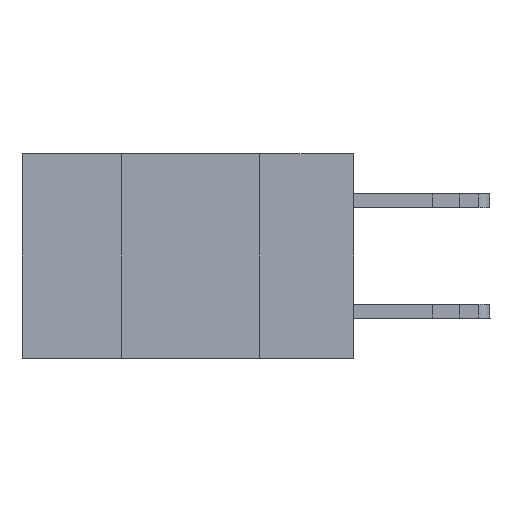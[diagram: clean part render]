
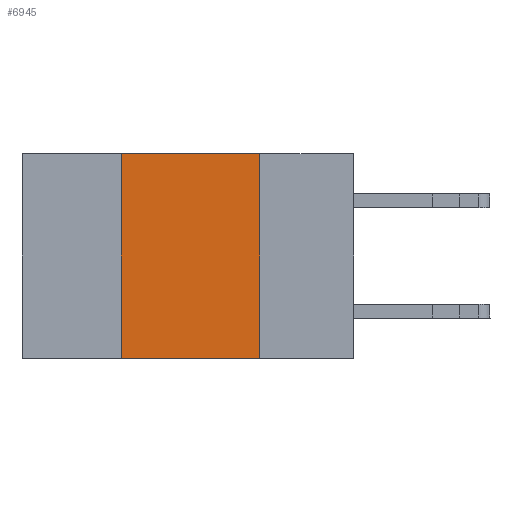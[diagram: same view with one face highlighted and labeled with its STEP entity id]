
A CAD part, left-side view. The second image highlights one B-rep face of the part: STEP entity #6945.
In plain terms, the highlighted planar face has unit normal (-1, 0, 0).
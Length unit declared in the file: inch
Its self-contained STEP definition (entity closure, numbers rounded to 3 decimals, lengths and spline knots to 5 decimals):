
#1055 = ORIENTED_EDGE ( 'NONE', *, *, #6135, .F. ) ;
#1481 = CARTESIAN_POINT ( 'NONE',  ( 0., 0.42, 0. ) ) ;
#1573 = DIRECTION ( 'NONE',  ( 0., 0., 1. ) ) ;
#2128 = DIRECTION ( 'NONE',  ( 0., 0., -1. ) ) ;
#2365 = PLANE ( 'NONE',  #15546 ) ;
#3663 = EDGE_CURVE ( 'NONE', #11657, #14002, #18799, .T. ) ;
#3861 = DIRECTION ( 'NONE',  ( 0., 0., -1. ) ) ;
#4919 = VERTEX_POINT ( 'NONE', #12031 ) ;
#6135 = EDGE_CURVE ( 'NONE', #14002, #4919, #16104, .T. ) ;
#6945 = ADVANCED_FACE ( 'NONE', ( #17276 ), #2365, .F. ) ;
#7197 = LINE ( 'NONE', #10608, #14643 ) ;
#7271 = ORIENTED_EDGE ( 'NONE', *, *, #3663, .F. ) ;
#7960 = VECTOR ( 'NONE', #16594, 39.37008 ) ;
#9075 = LINE ( 'NONE', #12852, #12044 ) ;
#9077 = EDGE_CURVE ( 'NONE', #13893, #11657, #7197, .T. ) ;
#9444 = EDGE_CURVE ( 'NONE', #13893, #4919, #9075, .T. ) ;
#9896 = DIRECTION ( 'NONE',  ( 0., -1., 0. ) ) ;
#10608 = CARTESIAN_POINT ( 'NONE',  ( 0., 0.42, 0. ) ) ;
#11132 = CARTESIAN_POINT ( 'NONE',  ( 0., 0.17, 0. ) ) ;
#11228 = VECTOR ( 'NONE', #2128, 39.37008 ) ;
#11385 = EDGE_LOOP ( 'NONE', ( #1055, #7271, #14712, #11914 ) ) ;
#11657 = VERTEX_POINT ( 'NONE', #1481 ) ;
#11914 = ORIENTED_EDGE ( 'NONE', *, *, #9444, .T. ) ;
#12031 = CARTESIAN_POINT ( 'NONE',  ( 0., 0.17, -0.37 ) ) ;
#12044 = VECTOR ( 'NONE', #9896, 39.37008 ) ;
#12844 = DIRECTION ( 'NONE',  ( 1., 0., 0. ) ) ;
#12852 = CARTESIAN_POINT ( 'NONE',  ( 0., 0.6, -0.37 ) ) ;
#13893 = VERTEX_POINT ( 'NONE', #16027 ) ;
#14002 = VERTEX_POINT ( 'NONE', #14793 ) ;
#14643 = VECTOR ( 'NONE', #1573, 39.37008 ) ;
#14712 = ORIENTED_EDGE ( 'NONE', *, *, #9077, .F. ) ;
#14793 = CARTESIAN_POINT ( 'NONE',  ( 0., 0.17, 0. ) ) ;
#15546 = AXIS2_PLACEMENT_3D ( 'NONE', #18739, #12844, #3861 ) ;
#15784 = CARTESIAN_POINT ( 'NONE',  ( 0., 0.6, 0. ) ) ;
#16027 = CARTESIAN_POINT ( 'NONE',  ( 0., 0.42, -0.37 ) ) ;
#16104 = LINE ( 'NONE', #11132, #11228 ) ;
#16594 = DIRECTION ( 'NONE',  ( 0., -1., 0. ) ) ;
#17276 = FACE_OUTER_BOUND ( 'NONE', #11385, .T. ) ;
#18739 = CARTESIAN_POINT ( 'NONE',  ( 0., 0.6, 0. ) ) ;
#18799 = LINE ( 'NONE', #15784, #7960 ) ;
